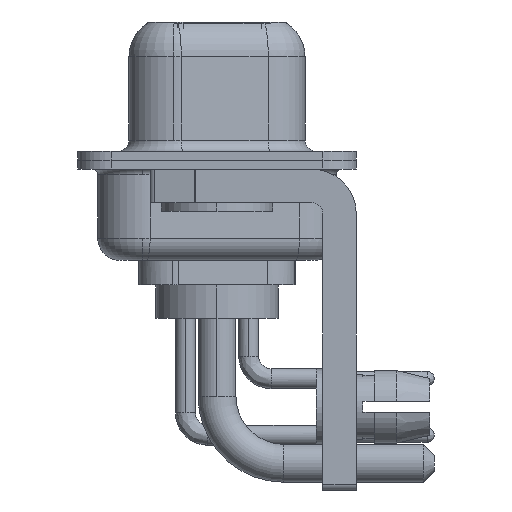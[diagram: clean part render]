
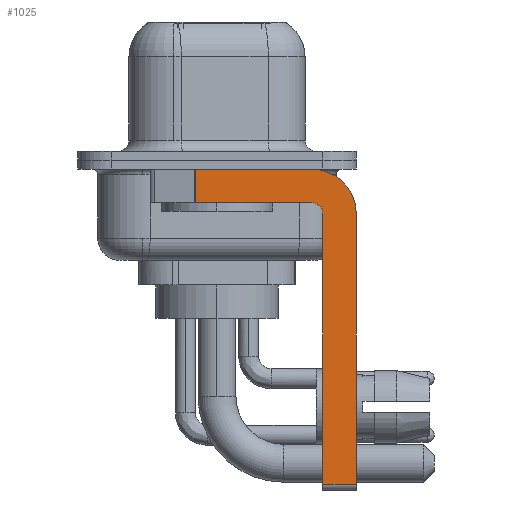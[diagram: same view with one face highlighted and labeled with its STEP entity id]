
A CAD part, left-side view. The second image highlights one B-rep face of the part: STEP entity #1025.
In plain terms, the highlighted planar face has unit normal (-1, 0, 0).
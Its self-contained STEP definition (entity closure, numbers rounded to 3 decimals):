
#22 = DIRECTION ( 'NONE',  ( 0., 0., -1. ) ) ;
#106 = ORIENTED_EDGE ( 'NONE', *, *, #2159, .T. ) ;
#670 = VERTEX_POINT ( 'NONE', #9081 ) ;
#1025 = ADVANCED_FACE ( 'NONE', ( #1713 ), #18370, .F. ) ;
#1713 = FACE_OUTER_BOUND ( 'NONE', #18945, .T. ) ;
#2025 = VECTOR ( 'NONE', #10602, 1000. ) ;
#2159 = EDGE_CURVE ( 'NONE', #670, #26885, #26076, .T. ) ;
#3084 = CARTESIAN_POINT ( 'NONE',  ( -2.9, -4.25, -14.55 ) ) ;
#4849 = ORIENTED_EDGE ( 'NONE', *, *, #11524, .T. ) ;
#4960 = CARTESIAN_POINT ( 'NONE',  ( -2.9, -4.25, -1.9 ) ) ;
#5187 = EDGE_CURVE ( 'NONE', #670, #23850, #14304, .T. ) ;
#5949 = CARTESIAN_POINT ( 'NONE',  ( -2.9, -6.25, -2.4 ) ) ;
#6077 = CARTESIAN_POINT ( 'NONE',  ( -2.9, -4.25, -1.9 ) ) ;
#6354 = CIRCLE ( 'NONE', #12960, 0.5 ) ;
#7465 = ORIENTED_EDGE ( 'NONE', *, *, #11887, .F. ) ;
#8113 = EDGE_CURVE ( 'NONE', #13327, #26885, #8154, .T. ) ;
#8154 = LINE ( 'NONE', #5949, #16961 ) ;
#8213 = EDGE_CURVE ( 'NONE', #23850, #12993, #6354, .T. ) ;
#8267 = LINE ( 'NONE', #23117, #17931 ) ;
#8427 = DIRECTION ( 'NONE',  ( -1., 0., 0. ) ) ;
#8662 = CARTESIAN_POINT ( 'NONE',  ( -2.9, -4.25, -0.4 ) ) ;
#9081 = CARTESIAN_POINT ( 'NONE',  ( -2.9, -4.75, -14.55 ) ) ;
#9762 = ORIENTED_EDGE ( 'NONE', *, *, #5187, .F. ) ;
#10326 = DIRECTION ( 'NONE',  ( 1., 0., 0. ) ) ;
#10486 = CARTESIAN_POINT ( 'NONE',  ( -2.9, -4.25, -2.4 ) ) ;
#10491 = CIRCLE ( 'NONE', #22788, 2. ) ;
#10602 = DIRECTION ( 'NONE',  ( 0., 1., 0. ) ) ;
#11204 = DIRECTION ( 'NONE',  ( 0., -1., 0. ) ) ;
#11524 = EDGE_CURVE ( 'NONE', #20468, #22703, #8267, .T. ) ;
#11887 = EDGE_CURVE ( 'NONE', #20468, #16577, #24471, .T. ) ;
#12133 = CARTESIAN_POINT ( 'NONE',  ( -2.9, -4.25, -2.4 ) ) ;
#12271 = DIRECTION ( 'NONE',  ( 0., 0., -1. ) ) ;
#12960 = AXIS2_PLACEMENT_3D ( 'NONE', #10486, #8427, #25616 ) ;
#12993 = VERTEX_POINT ( 'NONE', #4960 ) ;
#13327 = VERTEX_POINT ( 'NONE', #14973 ) ;
#13557 = CARTESIAN_POINT ( 'NONE',  ( -2.9, 0.978, -0.4 ) ) ;
#13765 = ORIENTED_EDGE ( 'NONE', *, *, #23455, .F. ) ;
#14112 = DIRECTION ( 'NONE',  ( 0., 0., -1. ) ) ;
#14158 = DIRECTION ( 'NONE',  ( 0., -1., 0. ) ) ;
#14304 = LINE ( 'NONE', #20628, #19826 ) ;
#14973 = CARTESIAN_POINT ( 'NONE',  ( -2.9, -6.25, -2.4 ) ) ;
#16577 = VERTEX_POINT ( 'NONE', #8662 ) ;
#16961 = VECTOR ( 'NONE', #22606, 1000. ) ;
#17931 = VECTOR ( 'NONE', #22, 1000. ) ;
#18370 = PLANE ( 'NONE',  #19059 ) ;
#18391 = VECTOR ( 'NONE', #14158, 1000. ) ;
#18945 = EDGE_LOOP ( 'NONE', ( #7465, #4849, #22738, #25330, #9762, #106, #19140, #13765 ) ) ;
#19059 = AXIS2_PLACEMENT_3D ( 'NONE', #22367, #26761, #14112 ) ;
#19090 = CARTESIAN_POINT ( 'NONE',  ( -2.9, 0.978, -1.9 ) ) ;
#19140 = ORIENTED_EDGE ( 'NONE', *, *, #8113, .F. ) ;
#19756 = EDGE_CURVE ( 'NONE', #12993, #22703, #26849, .T. ) ;
#19826 = VECTOR ( 'NONE', #25027, 1000. ) ;
#20468 = VERTEX_POINT ( 'NONE', #13557 ) ;
#20628 = CARTESIAN_POINT ( 'NONE',  ( -2.9, -4.75, -14.8 ) ) ;
#22367 = CARTESIAN_POINT ( 'NONE',  ( -2.9, -4.25, -2.4 ) ) ;
#22606 = DIRECTION ( 'NONE',  ( 0., 0., -1. ) ) ;
#22703 = VERTEX_POINT ( 'NONE', #19090 ) ;
#22738 = ORIENTED_EDGE ( 'NONE', *, *, #19756, .F. ) ;
#22788 = AXIS2_PLACEMENT_3D ( 'NONE', #12133, #10326, #12271 ) ;
#23117 = CARTESIAN_POINT ( 'NONE',  ( -2.9, 0.978, -1.9 ) ) ;
#23455 = EDGE_CURVE ( 'NONE', #16577, #13327, #10491, .T. ) ;
#23850 = VERTEX_POINT ( 'NONE', #24752 ) ;
#24471 = LINE ( 'NONE', #26807, #18391 ) ;
#24752 = CARTESIAN_POINT ( 'NONE',  ( -2.9, -4.75, -2.4 ) ) ;
#25027 = DIRECTION ( 'NONE',  ( 0., 0., 1. ) ) ;
#25330 = ORIENTED_EDGE ( 'NONE', *, *, #8213, .F. ) ;
#25616 = DIRECTION ( 'NONE',  ( 0., 0., 1. ) ) ;
#26076 = LINE ( 'NONE', #3084, #26535 ) ;
#26535 = VECTOR ( 'NONE', #11204, 1000. ) ;
#26761 = DIRECTION ( 'NONE',  ( 1., 0., 0. ) ) ;
#26807 = CARTESIAN_POINT ( 'NONE',  ( -2.9, 3., -0.4 ) ) ;
#26849 = LINE ( 'NONE', #6077, #2025 ) ;
#26885 = VERTEX_POINT ( 'NONE', #26919 ) ;
#26919 = CARTESIAN_POINT ( 'NONE',  ( -2.9, -6.25, -14.55 ) ) ;
